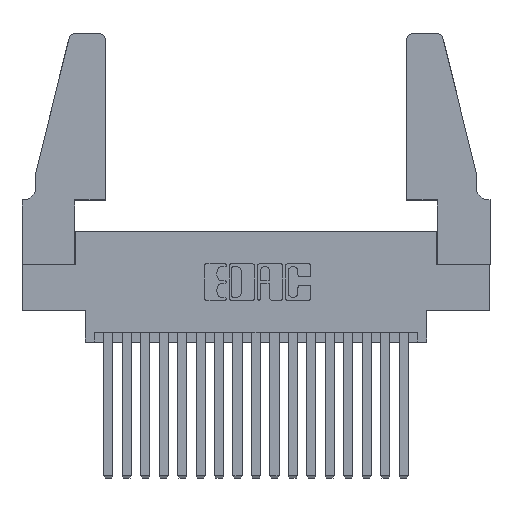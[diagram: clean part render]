
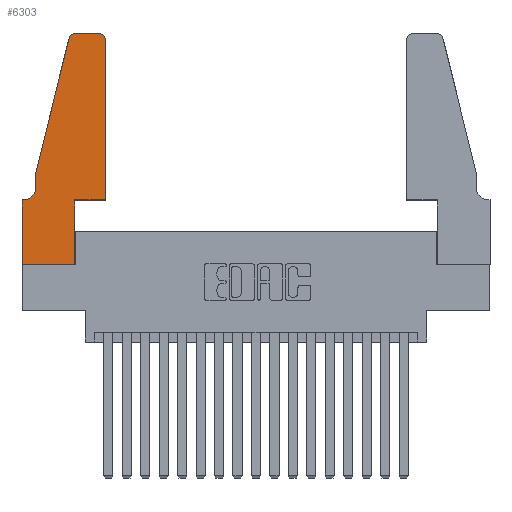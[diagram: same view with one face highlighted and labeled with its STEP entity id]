
A CAD part, top view. The second image highlights one B-rep face of the part: STEP entity #6303.
In plain terms, the highlighted planar face has unit normal (0, 0, 1).
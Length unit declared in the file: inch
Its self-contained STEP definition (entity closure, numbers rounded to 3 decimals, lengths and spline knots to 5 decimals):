
#109 = CARTESIAN_POINT ( 'NONE',  ( 0.284, 1.25, 0.37 ) ) ;
#325 = LINE ( 'NONE', #3599, #15392 ) ;
#467 = VERTEX_POINT ( 'NONE', #12377 ) ;
#490 = ORIENTED_EDGE ( 'NONE', *, *, #7779, .T. ) ;
#634 = DIRECTION ( 'NONE',  ( 0., -1., 0. ) ) ;
#638 = DIRECTION ( 'NONE',  ( -0.239, -0.971, 0. ) ) ;
#998 = DIRECTION ( 'NONE',  ( 0., -1., 0. ) ) ;
#1865 = VERTEX_POINT ( 'NONE', #9329 ) ;
#2151 = ORIENTED_EDGE ( 'NONE', *, *, #14216, .T. ) ;
#2173 = ORIENTED_EDGE ( 'NONE', *, *, #14493, .T. ) ;
#2215 = ORIENTED_EDGE ( 'NONE', *, *, #15372, .T. ) ;
#2248 = VERTEX_POINT ( 'NONE', #13017 ) ;
#2295 = ORIENTED_EDGE ( 'NONE', *, *, #9410, .T. ) ;
#2314 = ORIENTED_EDGE ( 'NONE', *, *, #9822, .T. ) ;
#2382 = CARTESIAN_POINT ( 'NONE',  ( 0.4205, 1.22, 0.37 ) ) ;
#2452 = CARTESIAN_POINT ( 'NONE',  ( 0.0755, 0.5, 0.37 ) ) ;
#2761 = LINE ( 'NONE', #17292, #17186 ) ;
#2765 = DIRECTION ( 'NONE',  ( 0., 1., 0. ) ) ;
#2831 = LINE ( 'NONE', #12213, #10548 ) ;
#3099 = CARTESIAN_POINT ( 'NONE',  ( 0.284, 1.22, 0.37 ) ) ;
#3165 = EDGE_CURVE ( 'NONE', #467, #6517, #4202, .T. ) ;
#3507 = LINE ( 'NONE', #17539, #10777 ) ;
#3599 = CARTESIAN_POINT ( 'NONE',  ( 0.0755, 0.5, 0.37 ) ) ;
#3726 = PLANE ( 'NONE',  #13125 ) ;
#3771 = LINE ( 'NONE', #9451, #14854 ) ;
#3868 = LINE ( 'NONE', #13475, #7719 ) ;
#3880 = DIRECTION ( 'NONE',  ( 1., 0., 0. ) ) ;
#4013 = CIRCLE ( 'NONE', #12912, 0.03 ) ;
#4072 = DIRECTION ( 'NONE',  ( -1., 0., 0. ) ) ;
#4202 = CIRCLE ( 'NONE', #5721, 0.07 ) ;
#4334 = AXIS2_PLACEMENT_3D ( 'NONE', #2382, #12540, #3880 ) ;
#4413 = VERTEX_POINT ( 'NONE', #9245 ) ;
#4585 = DIRECTION ( 'NONE',  ( 1., 0., 0. ) ) ;
#4948 = ORIENTED_EDGE ( 'NONE', *, *, #10372, .T. ) ;
#5000 = CARTESIAN_POINT ( 'NONE',  ( 0.25487, 1.22718, 0.37 ) ) ;
#5104 = DIRECTION ( 'NONE',  ( 0., 0., -1. ) ) ;
#5721 = AXIS2_PLACEMENT_3D ( 'NONE', #13747, #5104, #15191 ) ;
#5777 = VERTEX_POINT ( 'NONE', #13938 ) ;
#6104 = DIRECTION ( 'NONE',  ( 1., 0., 0. ) ) ;
#6264 = DIRECTION ( 'NONE',  ( -1., 0., 0. ) ) ;
#6303 = ADVANCED_FACE ( 'NONE', ( #9964 ), #3726, .T. ) ;
#6517 = VERTEX_POINT ( 'NONE', #14225 ) ;
#6645 = DIRECTION ( 'NONE',  ( 1., 0., 0. ) ) ;
#7155 = CARTESIAN_POINT ( 'NONE',  ( 0.2865, 0.35, 0.37 ) ) ;
#7253 = DIRECTION ( 'NONE',  ( 0., 1., 0. ) ) ;
#7641 = LINE ( 'NONE', #12723, #15769 ) ;
#7719 = VECTOR ( 'NONE', #6264, 39.37008 ) ;
#7779 = EDGE_CURVE ( 'NONE', #10329, #467, #15747, .T. ) ;
#7856 = CARTESIAN_POINT ( 'NONE',  ( 0.0755, 0.5, 0.37 ) ) ;
#7871 = ORIENTED_EDGE ( 'NONE', *, *, #3165, .T. ) ;
#8067 = EDGE_CURVE ( 'NONE', #1865, #11116, #7641, .T. ) ;
#8303 = EDGE_CURVE ( 'NONE', #11116, #16717, #4013, .T. ) ;
#8543 = EDGE_CURVE ( 'NONE', #15621, #5777, #3771, .T. ) ;
#8807 = ORIENTED_EDGE ( 'NONE', *, *, #8303, .T. ) ;
#9245 = CARTESIAN_POINT ( 'NONE',  ( 0.2865, 0., 0.37 ) ) ;
#9329 = CARTESIAN_POINT ( 'NONE',  ( 0.4205, 1.25, 0.37 ) ) ;
#9410 = EDGE_CURVE ( 'NONE', #10429, #2248, #2761, .T. ) ;
#9422 = VECTOR ( 'NONE', #2765, 39.37008 ) ;
#9451 = CARTESIAN_POINT ( 'NONE',  ( 0., 0., 0.37 ) ) ;
#9516 = CARTESIAN_POINT ( 'NONE',  ( 0., 0.35, 0.37 ) ) ;
#9822 = EDGE_CURVE ( 'NONE', #2248, #1865, #10476, .T. ) ;
#9964 = FACE_OUTER_BOUND ( 'NONE', #15057, .T. ) ;
#10329 = VERTEX_POINT ( 'NONE', #7856 ) ;
#10372 = EDGE_CURVE ( 'NONE', #16717, #10329, #325, .T. ) ;
#10429 = VERTEX_POINT ( 'NONE', #13852 ) ;
#10476 = CIRCLE ( 'NONE', #4334, 0.03 ) ;
#10548 = VECTOR ( 'NONE', #10837, 39.37008 ) ;
#10619 = CARTESIAN_POINT ( 'NONE',  ( 0.2865, 0.35, 0.37 ) ) ;
#10777 = VECTOR ( 'NONE', #6104, 39.37008 ) ;
#10837 = DIRECTION ( 'NONE',  ( 1., 0., 0. ) ) ;
#11116 = VERTEX_POINT ( 'NONE', #109 ) ;
#11922 = VECTOR ( 'NONE', #998, 39.37008 ) ;
#12213 = CARTESIAN_POINT ( 'NONE',  ( 0., 0., 0.37 ) ) ;
#12377 = CARTESIAN_POINT ( 'NONE',  ( 0.0755, 0.42, 0.37 ) ) ;
#12416 = CARTESIAN_POINT ( 'NONE',  ( 0., 0.35, 0.37 ) ) ;
#12540 = DIRECTION ( 'NONE',  ( 0., 0., 1. ) ) ;
#12601 = VERTEX_POINT ( 'NONE', #10619 ) ;
#12723 = CARTESIAN_POINT ( 'NONE',  ( 0.2605, 1.25, 0.37 ) ) ;
#12912 = AXIS2_PLACEMENT_3D ( 'NONE', #3099, #13227, #4585 ) ;
#13017 = CARTESIAN_POINT ( 'NONE',  ( 0.4505, 1.22, 0.37 ) ) ;
#13069 = ORIENTED_EDGE ( 'NONE', *, *, #18581, .T. ) ;
#13125 = AXIS2_PLACEMENT_3D ( 'NONE', #9516, #15297, #6645 ) ;
#13227 = DIRECTION ( 'NONE',  ( 0., 0., 1. ) ) ;
#13475 = CARTESIAN_POINT ( 'NONE',  ( 0.0755, 0.35, 0.37 ) ) ;
#13747 = CARTESIAN_POINT ( 'NONE',  ( 0.0055, 0.42, 0.37 ) ) ;
#13852 = CARTESIAN_POINT ( 'NONE',  ( 0.4505, 0.35, 0.37 ) ) ;
#13938 = CARTESIAN_POINT ( 'NONE',  ( 0., 0., 0.37 ) ) ;
#14216 = EDGE_CURVE ( 'NONE', #5777, #4413, #2831, .T. ) ;
#14225 = CARTESIAN_POINT ( 'NONE',  ( 0.0055, 0.35, 0.37 ) ) ;
#14493 = EDGE_CURVE ( 'NONE', #4413, #12601, #17019, .T. ) ;
#14854 = VECTOR ( 'NONE', #634, 39.37008 ) ;
#15057 = EDGE_LOOP ( 'NONE', ( #18431, #8807, #4948, #490, #7871, #13069, #16867, #2151, #2173, #2215, #2295, #2314 ) ) ;
#15191 = DIRECTION ( 'NONE',  ( -1., 0., 0. ) ) ;
#15297 = DIRECTION ( 'NONE',  ( 0., 0., 1. ) ) ;
#15372 = EDGE_CURVE ( 'NONE', #12601, #10429, #3507, .T. ) ;
#15392 = VECTOR ( 'NONE', #638, 39.37008 ) ;
#15621 = VERTEX_POINT ( 'NONE', #12416 ) ;
#15747 = LINE ( 'NONE', #2452, #11922 ) ;
#15769 = VECTOR ( 'NONE', #4072, 39.37008 ) ;
#16717 = VERTEX_POINT ( 'NONE', #5000 ) ;
#16867 = ORIENTED_EDGE ( 'NONE', *, *, #8543, .T. ) ;
#17019 = LINE ( 'NONE', #7155, #9422 ) ;
#17186 = VECTOR ( 'NONE', #7253, 39.37008 ) ;
#17292 = CARTESIAN_POINT ( 'NONE',  ( 0.4505, 0.35, 0.37 ) ) ;
#17539 = CARTESIAN_POINT ( 'NONE',  ( 0.4505, 0.35, 0.37 ) ) ;
#18431 = ORIENTED_EDGE ( 'NONE', *, *, #8067, .T. ) ;
#18581 = EDGE_CURVE ( 'NONE', #6517, #15621, #3868, .T. ) ;
